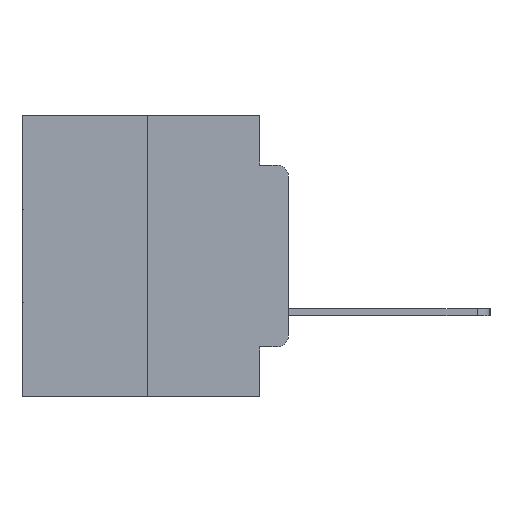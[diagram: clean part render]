
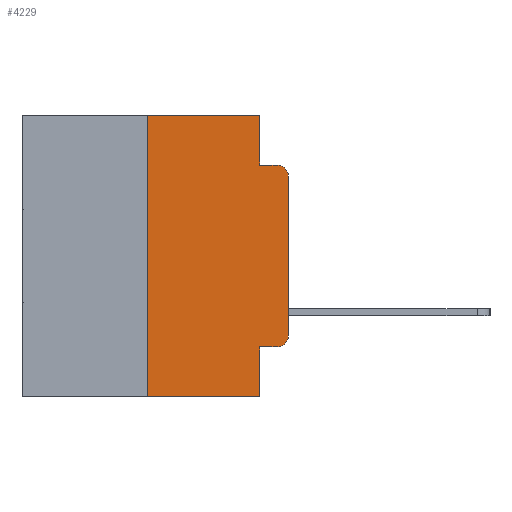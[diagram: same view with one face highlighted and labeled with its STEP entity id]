
A CAD part, left-side view. The second image highlights one B-rep face of the part: STEP entity #4229.
In plain terms, the highlighted planar face has unit normal (-1, 0, 0).
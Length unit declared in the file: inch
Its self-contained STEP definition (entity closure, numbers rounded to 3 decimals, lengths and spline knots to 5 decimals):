
#157 = DIRECTION ( 'NONE',  ( 0., 0., -1. ) ) ;
#172 = EDGE_CURVE ( 'NONE', #4068, #25625, #25172, .T. ) ;
#599 = DIRECTION ( 'NONE',  ( 0., 0., -1. ) ) ;
#1727 = VECTOR ( 'NONE', #19529, 39.37008 ) ;
#2205 = VECTOR ( 'NONE', #25096, 39.37008 ) ;
#2365 = CARTESIAN_POINT ( 'NONE',  ( 0., 0.051, -0.4115 ) ) ;
#2448 = VERTEX_POINT ( 'NONE', #8283 ) ;
#2495 = CARTESIAN_POINT ( 'NONE',  ( 0., 0.051, -0.0885 ) ) ;
#2775 = ORIENTED_EDGE ( 'NONE', *, *, #23075, .T. ) ;
#2831 = VECTOR ( 'NONE', #11326, 39.37008 ) ;
#2908 = VECTOR ( 'NONE', #21648, 39.37008 ) ;
#3104 = ORIENTED_EDGE ( 'NONE', *, *, #12084, .F. ) ;
#4068 = VERTEX_POINT ( 'NONE', #8358 ) ;
#4087 = EDGE_CURVE ( 'NONE', #2448, #4068, #7452, .T. ) ;
#4160 = VERTEX_POINT ( 'NONE', #4311 ) ;
#4229 = ADVANCED_FACE ( 'NONE', ( #4331 ), #23478, .F. ) ;
#4311 = CARTESIAN_POINT ( 'NONE',  ( 0., 0.25, -0.5 ) ) ;
#4331 = FACE_OUTER_BOUND ( 'NONE', #8300, .T. ) ;
#4364 = AXIS2_PLACEMENT_3D ( 'NONE', #25515, #13384, #157 ) ;
#4602 = DIRECTION ( 'NONE',  ( 0., 0., -1. ) ) ;
#4734 = EDGE_CURVE ( 'NONE', #4160, #8907, #14559, .T. ) ;
#4791 = DIRECTION ( 'NONE',  ( -1., 0., 0. ) ) ;
#5122 = LINE ( 'NONE', #25303, #26657 ) ;
#5208 = ORIENTED_EDGE ( 'NONE', *, *, #17628, .F. ) ;
#5910 = CARTESIAN_POINT ( 'NONE',  ( 0., 0.051, -0.4115 ) ) ;
#7358 = ORIENTED_EDGE ( 'NONE', *, *, #4087, .T. ) ;
#7452 = LINE ( 'NONE', #10641, #23419 ) ;
#7675 = LINE ( 'NONE', #2365, #1727 ) ;
#8278 = VERTEX_POINT ( 'NONE', #24965 ) ;
#8283 = CARTESIAN_POINT ( 'NONE',  ( 0., 0., -0.3915 ) ) ;
#8300 = EDGE_LOOP ( 'NONE', ( #7358, #18614, #3104, #14745, #10432, #5208, #17921, #23312, #2775, #25792 ) ) ;
#8358 = CARTESIAN_POINT ( 'NONE',  ( 0., 0., -0.1085 ) ) ;
#8486 = VECTOR ( 'NONE', #25855, 39.37008 ) ;
#8907 = VERTEX_POINT ( 'NONE', #11246 ) ;
#9018 = CARTESIAN_POINT ( 'NONE',  ( 0., 0.473, 0. ) ) ;
#9230 = CARTESIAN_POINT ( 'NONE',  ( 0., 0.473, 0. ) ) ;
#10432 = ORIENTED_EDGE ( 'NONE', *, *, #18323, .F. ) ;
#10641 = CARTESIAN_POINT ( 'NONE',  ( 0., 0., 0. ) ) ;
#11246 = CARTESIAN_POINT ( 'NONE',  ( 0., 0.051, -0.5 ) ) ;
#11326 = DIRECTION ( 'NONE',  ( 0., 0., -1. ) ) ;
#12084 = EDGE_CURVE ( 'NONE', #19035, #25625, #24947, .T. ) ;
#12419 = CARTESIAN_POINT ( 'NONE',  ( 0., 0.02, -0.1085 ) ) ;
#12974 = LINE ( 'NONE', #25851, #23784 ) ;
#13162 = DIRECTION ( 'NONE',  ( 0., 0., -1. ) ) ;
#13384 = DIRECTION ( 'NONE',  ( -1., 0., 0. ) ) ;
#13731 = DIRECTION ( 'NONE',  ( 0., 0., 1. ) ) ;
#14489 = LINE ( 'NONE', #21587, #2831 ) ;
#14559 = LINE ( 'NONE', #23118, #2205 ) ;
#14570 = LINE ( 'NONE', #9230, #2908 ) ;
#14745 = ORIENTED_EDGE ( 'NONE', *, *, #16270, .F. ) ;
#15828 = CARTESIAN_POINT ( 'NONE',  ( 0., 0.051, -0.0885 ) ) ;
#16270 = EDGE_CURVE ( 'NONE', #22847, #19035, #5122, .T. ) ;
#17473 = DIRECTION ( 'NONE',  ( 1., 0., 0. ) ) ;
#17628 = EDGE_CURVE ( 'NONE', #4160, #8278, #12974, .T. ) ;
#17921 = ORIENTED_EDGE ( 'NONE', *, *, #4734, .T. ) ;
#18263 = VERTEX_POINT ( 'NONE', #25476 ) ;
#18323 = EDGE_CURVE ( 'NONE', #8278, #22847, #14570, .T. ) ;
#18614 = ORIENTED_EDGE ( 'NONE', *, *, #172, .T. ) ;
#19035 = VERTEX_POINT ( 'NONE', #2495 ) ;
#19174 = AXIS2_PLACEMENT_3D ( 'NONE', #9018, #17473, #4602 ) ;
#19529 = DIRECTION ( 'NONE',  ( 0., -1., 0. ) ) ;
#20864 = DIRECTION ( 'NONE',  ( 0., 0., 1. ) ) ;
#20963 = CARTESIAN_POINT ( 'NONE',  ( 0., 0.051, 0. ) ) ;
#21332 = VERTEX_POINT ( 'NONE', #5910 ) ;
#21587 = CARTESIAN_POINT ( 'NONE',  ( 0., 0.051, 0. ) ) ;
#21648 = DIRECTION ( 'NONE',  ( 0., -1., 0. ) ) ;
#21702 = EDGE_CURVE ( 'NONE', #21332, #8907, #14489, .T. ) ;
#22847 = VERTEX_POINT ( 'NONE', #20963 ) ;
#23075 = EDGE_CURVE ( 'NONE', #21332, #18263, #7675, .T. ) ;
#23118 = CARTESIAN_POINT ( 'NONE',  ( 0., 0.473, -0.5 ) ) ;
#23312 = ORIENTED_EDGE ( 'NONE', *, *, #21702, .F. ) ;
#23419 = VECTOR ( 'NONE', #20864, 39.37008 ) ;
#23478 = PLANE ( 'NONE',  #19174 ) ;
#23784 = VECTOR ( 'NONE', #13731, 39.37008 ) ;
#24947 = LINE ( 'NONE', #15828, #8486 ) ;
#24965 = CARTESIAN_POINT ( 'NONE',  ( 0., 0.25, 0. ) ) ;
#25096 = DIRECTION ( 'NONE',  ( 0., -1., 0. ) ) ;
#25172 = CIRCLE ( 'NONE', #26966, 0.02 ) ;
#25269 = CARTESIAN_POINT ( 'NONE',  ( 0., 0.02, -0.0885 ) ) ;
#25303 = CARTESIAN_POINT ( 'NONE',  ( 0., 0.051, 0. ) ) ;
#25476 = CARTESIAN_POINT ( 'NONE',  ( 0., 0.02, -0.4115 ) ) ;
#25515 = CARTESIAN_POINT ( 'NONE',  ( 0., 0.02, -0.3915 ) ) ;
#25625 = VERTEX_POINT ( 'NONE', #25269 ) ;
#25702 = EDGE_CURVE ( 'NONE', #18263, #2448, #26451, .T. ) ;
#25792 = ORIENTED_EDGE ( 'NONE', *, *, #25702, .T. ) ;
#25851 = CARTESIAN_POINT ( 'NONE',  ( 0., 0.25, 0. ) ) ;
#25855 = DIRECTION ( 'NONE',  ( 0., -1., 0. ) ) ;
#26451 = CIRCLE ( 'NONE', #4364, 0.02 ) ;
#26657 = VECTOR ( 'NONE', #13162, 39.37008 ) ;
#26966 = AXIS2_PLACEMENT_3D ( 'NONE', #12419, #4791, #599 ) ;
